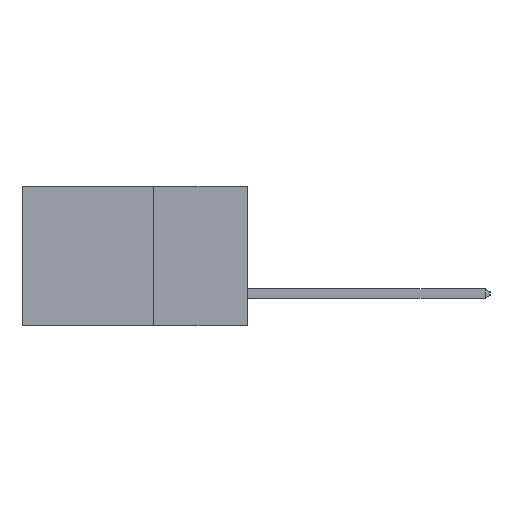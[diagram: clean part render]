
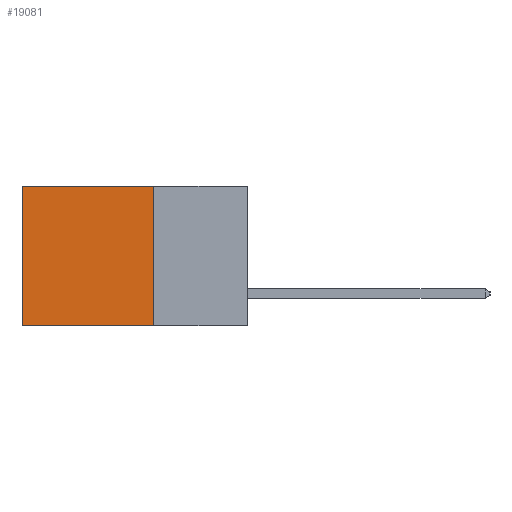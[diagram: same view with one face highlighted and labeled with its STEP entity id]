
A CAD part, left-side view. The second image highlights one B-rep face of the part: STEP entity #19081.
In plain terms, the highlighted planar face has unit normal (-1, 0, 0).
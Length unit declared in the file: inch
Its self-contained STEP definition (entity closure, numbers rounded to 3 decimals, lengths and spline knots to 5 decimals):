
#480 = ORIENTED_EDGE ( 'NONE', *, *, #19466, .T. ) ;
#852 = CARTESIAN_POINT ( 'NONE',  ( 0.2615, 0.6, -0.37 ) ) ;
#2091 = CARTESIAN_POINT ( 'NONE',  ( 0.2615, 0.25, -0.37 ) ) ;
#2254 = CARTESIAN_POINT ( 'NONE',  ( 0.2615, 0.25, -0.37 ) ) ;
#2578 = VECTOR ( 'NONE', #8964, 39.37008 ) ;
#2900 = EDGE_LOOP ( 'NONE', ( #12552, #9502, #18782, #480 ) ) ;
#3136 = AXIS2_PLACEMENT_3D ( 'NONE', #2091, #12994, #3628 ) ;
#3327 = LINE ( 'NONE', #13795, #3806 ) ;
#3605 = VERTEX_POINT ( 'NONE', #11467 ) ;
#3628 = DIRECTION ( 'NONE',  ( 0., 0., -1. ) ) ;
#3806 = VECTOR ( 'NONE', #13735, 39.37008 ) ;
#4278 = LINE ( 'NONE', #2254, #7913 ) ;
#7759 = EDGE_CURVE ( 'NONE', #3605, #17094, #3327, .T. ) ;
#7913 = VECTOR ( 'NONE', #11613, 39.37008 ) ;
#7925 = VECTOR ( 'NONE', #19859, 39.37008 ) ;
#8408 = EDGE_CURVE ( 'NONE', #16649, #14068, #18996, .T. ) ;
#8421 = LINE ( 'NONE', #18359, #7925 ) ;
#8560 = CARTESIAN_POINT ( 'NONE',  ( 0.2615, 0.6, 0. ) ) ;
#8964 = DIRECTION ( 'NONE',  ( 0., 0., -1. ) ) ;
#9502 = ORIENTED_EDGE ( 'NONE', *, *, #19855, .F. ) ;
#10078 = CARTESIAN_POINT ( 'NONE',  ( 0.2615, 0.6, -0.37 ) ) ;
#11467 = CARTESIAN_POINT ( 'NONE',  ( 0.2615, 0.25, 0. ) ) ;
#11613 = DIRECTION ( 'NONE',  ( 0., 1., 0. ) ) ;
#12552 = ORIENTED_EDGE ( 'NONE', *, *, #8408, .T. ) ;
#12916 = PLANE ( 'NONE',  #3136 ) ;
#12994 = DIRECTION ( 'NONE',  ( 1., 0., 0. ) ) ;
#13735 = DIRECTION ( 'NONE',  ( 0., 0., -1. ) ) ;
#13795 = CARTESIAN_POINT ( 'NONE',  ( 0.2615, 0.25, -0.37 ) ) ;
#14068 = VERTEX_POINT ( 'NONE', #852 ) ;
#15239 = FACE_OUTER_BOUND ( 'NONE', #2900, .T. ) ;
#16649 = VERTEX_POINT ( 'NONE', #8560 ) ;
#17094 = VERTEX_POINT ( 'NONE', #17651 ) ;
#17651 = CARTESIAN_POINT ( 'NONE',  ( 0.2615, 0.25, -0.37 ) ) ;
#18359 = CARTESIAN_POINT ( 'NONE',  ( 0.2615, 0.25, 0. ) ) ;
#18782 = ORIENTED_EDGE ( 'NONE', *, *, #7759, .F. ) ;
#18996 = LINE ( 'NONE', #10078, #2578 ) ;
#19081 = ADVANCED_FACE ( 'NONE', ( #15239 ), #12916, .F. ) ;
#19466 = EDGE_CURVE ( 'NONE', #3605, #16649, #8421, .T. ) ;
#19855 = EDGE_CURVE ( 'NONE', #17094, #14068, #4278, .T. ) ;
#19859 = DIRECTION ( 'NONE',  ( 0., 1., 0. ) ) ;
